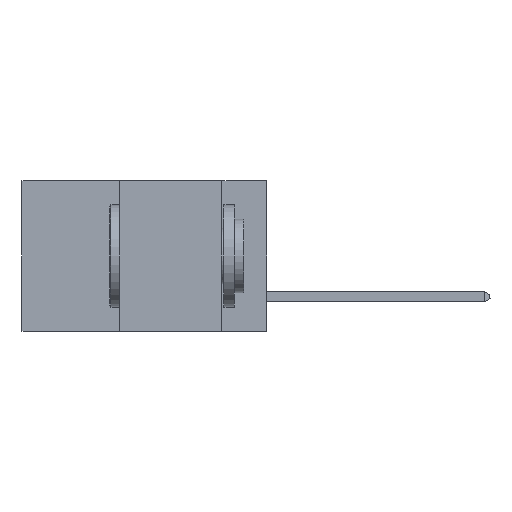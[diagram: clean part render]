
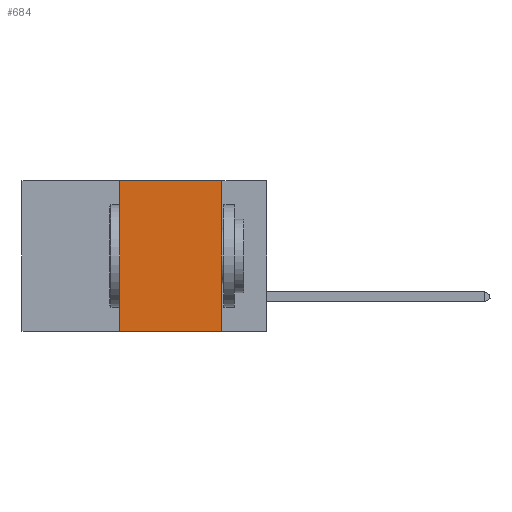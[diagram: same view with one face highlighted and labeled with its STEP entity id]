
A CAD part, left-side view. The second image highlights one B-rep face of the part: STEP entity #684.
In plain terms, the highlighted planar face has unit normal (-1, 0, 0).
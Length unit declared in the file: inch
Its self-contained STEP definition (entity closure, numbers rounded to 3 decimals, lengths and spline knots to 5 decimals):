
#342 = VERTEX_POINT ( 'NONE', #8817 ) ;
#484 = VERTEX_POINT ( 'NONE', #9029 ) ;
#631 = ORIENTED_EDGE ( 'NONE', *, *, #4407, .F. ) ;
#684 = ADVANCED_FACE ( 'NONE', ( #10684 ), #5011, .F. ) ;
#1270 = DIRECTION ( 'NONE',  ( 0., 0., -1. ) ) ;
#1371 = VECTOR ( 'NONE', #1752, 39.37008 ) ;
#1405 = CARTESIAN_POINT ( 'NONE',  ( 0., 0.6, 0. ) ) ;
#1487 = CARTESIAN_POINT ( 'NONE',  ( 0., 0.11, 0. ) ) ;
#1752 = DIRECTION ( 'NONE',  ( 0., 0., 1. ) ) ;
#1877 = ORIENTED_EDGE ( 'NONE', *, *, #3037, .F. ) ;
#2255 = LINE ( 'NONE', #1405, #10446 ) ;
#2635 = VERTEX_POINT ( 'NONE', #8688 ) ;
#3037 = EDGE_CURVE ( 'NONE', #5019, #342, #7646, .T. ) ;
#3081 = AXIS2_PLACEMENT_3D ( 'NONE', #5091, #10091, #8372 ) ;
#4195 = VECTOR ( 'NONE', #6712, 39.37008 ) ;
#4225 = EDGE_LOOP ( 'NONE', ( #1877, #10398, #631, #5391 ) ) ;
#4407 = EDGE_CURVE ( 'NONE', #2635, #484, #7999, .T. ) ;
#5011 = PLANE ( 'NONE',  #3081 ) ;
#5019 = VERTEX_POINT ( 'NONE', #1487 ) ;
#5091 = CARTESIAN_POINT ( 'NONE',  ( 0., 0.6, 0. ) ) ;
#5391 = ORIENTED_EDGE ( 'NONE', *, *, #7144, .T. ) ;
#5442 = CARTESIAN_POINT ( 'NONE',  ( 0., 0.11, 0. ) ) ;
#5803 = VECTOR ( 'NONE', #1270, 39.37008 ) ;
#5886 = CARTESIAN_POINT ( 'NONE',  ( 0., 0.36, 0. ) ) ;
#6311 = DIRECTION ( 'NONE',  ( 0., -1., 0. ) ) ;
#6712 = DIRECTION ( 'NONE',  ( 0., -1., 0. ) ) ;
#6757 = EDGE_CURVE ( 'NONE', #484, #5019, #2255, .T. ) ;
#7144 = EDGE_CURVE ( 'NONE', #2635, #342, #10701, .T. ) ;
#7512 = CARTESIAN_POINT ( 'NONE',  ( 0., 0.6, -0.37 ) ) ;
#7646 = LINE ( 'NONE', #5442, #5803 ) ;
#7999 = LINE ( 'NONE', #5886, #1371 ) ;
#8372 = DIRECTION ( 'NONE',  ( 0., 0., -1. ) ) ;
#8688 = CARTESIAN_POINT ( 'NONE',  ( 0., 0.36, -0.37 ) ) ;
#8817 = CARTESIAN_POINT ( 'NONE',  ( 0., 0.11, -0.37 ) ) ;
#9029 = CARTESIAN_POINT ( 'NONE',  ( 0., 0.36, 0. ) ) ;
#10091 = DIRECTION ( 'NONE',  ( 1., 0., 0. ) ) ;
#10398 = ORIENTED_EDGE ( 'NONE', *, *, #6757, .F. ) ;
#10446 = VECTOR ( 'NONE', #6311, 39.37008 ) ;
#10684 = FACE_OUTER_BOUND ( 'NONE', #4225, .T. ) ;
#10701 = LINE ( 'NONE', #7512, #4195 ) ;
